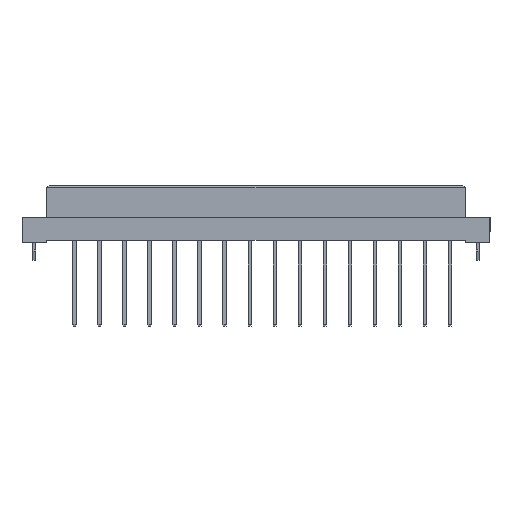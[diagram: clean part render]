
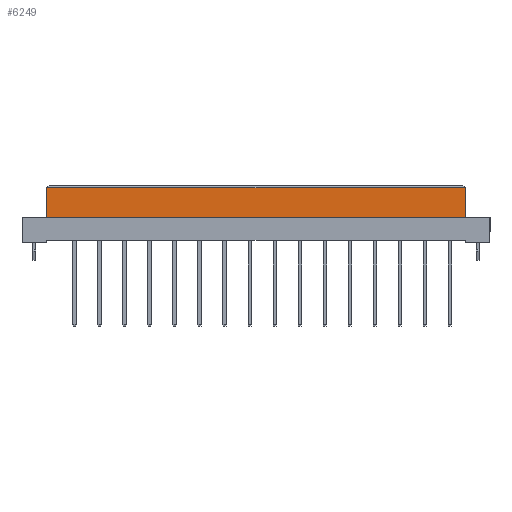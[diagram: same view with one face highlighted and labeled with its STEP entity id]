
A CAD part, top view. The second image highlights one B-rep face of the part: STEP entity #6249.
In plain terms, the highlighted planar face has unit normal (0, 0, 1).
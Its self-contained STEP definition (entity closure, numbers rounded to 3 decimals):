
#81 = CARTESIAN_POINT ( 'NONE',  ( -42.5, -6.4, 4.25 ) ) ;
#122 = CARTESIAN_POINT ( 'NONE',  ( -42.5, -0.5, 4.25 ) ) ;
#1637 = CARTESIAN_POINT ( 'NONE',  ( 42.5, -6.4, 4.25 ) ) ;
#2477 = LINE ( 'NONE', #81, #21821 ) ;
#3269 = DIRECTION ( 'NONE',  ( 0., 1., 0. ) ) ;
#3388 = CARTESIAN_POINT ( 'NONE',  ( 42.5, -6.4, 4.25 ) ) ;
#4199 = LINE ( 'NONE', #25141, #21241 ) ;
#6249 = ADVANCED_FACE ( 'NONE', ( #13480 ), #25640, .T. ) ;
#6381 = DIRECTION ( 'NONE',  ( 1., 0., 0. ) ) ;
#7029 = EDGE_LOOP ( 'NONE', ( #27115, #38858, #7597, #21436 ) ) ;
#7597 = ORIENTED_EDGE ( 'NONE', *, *, #9092, .F. ) ;
#8112 = DIRECTION ( 'NONE',  ( 0., 0., 1. ) ) ;
#8336 = CARTESIAN_POINT ( 'NONE',  ( -42.5, -6.4, 4.25 ) ) ;
#9092 = EDGE_CURVE ( 'NONE', #37528, #21990, #2477, .T. ) ;
#9982 = DIRECTION ( 'NONE',  ( 0., 1., 0. ) ) ;
#10846 = EDGE_CURVE ( 'NONE', #15531, #12817, #4199, .T. ) ;
#12817 = VERTEX_POINT ( 'NONE', #16415 ) ;
#13480 = FACE_OUTER_BOUND ( 'NONE', #7029, .T. ) ;
#15531 = VERTEX_POINT ( 'NONE', #1637 ) ;
#15733 = EDGE_CURVE ( 'NONE', #37528, #15531, #37281, .T. ) ;
#16415 = CARTESIAN_POINT ( 'NONE',  ( 42.5, -0.5, 4.25 ) ) ;
#17125 = AXIS2_PLACEMENT_3D ( 'NONE', #38018, #8112, #22661 ) ;
#21044 = LINE ( 'NONE', #122, #35196 ) ;
#21241 = VECTOR ( 'NONE', #9982, 1000. ) ;
#21247 = DIRECTION ( 'NONE',  ( -1., 0., 0. ) ) ;
#21436 = ORIENTED_EDGE ( 'NONE', *, *, #15733, .T. ) ;
#21821 = VECTOR ( 'NONE', #3269, 1000. ) ;
#21990 = VERTEX_POINT ( 'NONE', #25808 ) ;
#22661 = DIRECTION ( 'NONE',  ( 1., 0., 0. ) ) ;
#24606 = EDGE_CURVE ( 'NONE', #12817, #21990, #21044, .T. ) ;
#25141 = CARTESIAN_POINT ( 'NONE',  ( 42.5, -6.4, 4.25 ) ) ;
#25640 = PLANE ( 'NONE',  #17125 ) ;
#25808 = CARTESIAN_POINT ( 'NONE',  ( -42.5, -0.5, 4.25 ) ) ;
#27115 = ORIENTED_EDGE ( 'NONE', *, *, #10846, .T. ) ;
#35196 = VECTOR ( 'NONE', #21247, 1000. ) ;
#36773 = VECTOR ( 'NONE', #6381, 1000. ) ;
#37281 = LINE ( 'NONE', #3388, #36773 ) ;
#37528 = VERTEX_POINT ( 'NONE', #8336 ) ;
#38018 = CARTESIAN_POINT ( 'NONE',  ( 42.5, -6.4, 4.25 ) ) ;
#38858 = ORIENTED_EDGE ( 'NONE', *, *, #24606, .T. ) ;
